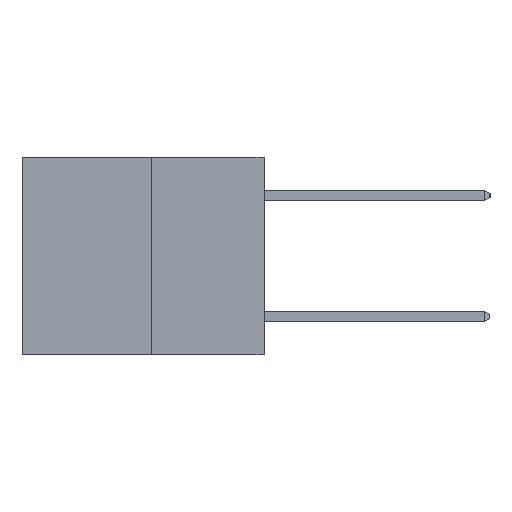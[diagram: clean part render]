
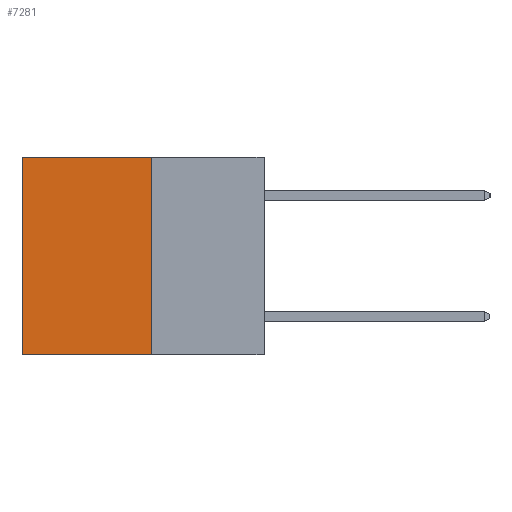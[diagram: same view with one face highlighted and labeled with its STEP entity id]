
A CAD part, left-side view. The second image highlights one B-rep face of the part: STEP entity #7281.
In plain terms, the highlighted planar face has unit normal (-1, 0, 0).
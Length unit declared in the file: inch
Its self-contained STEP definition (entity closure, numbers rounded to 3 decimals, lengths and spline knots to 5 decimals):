
#185 = CARTESIAN_POINT ( 'NONE',  ( 0.3165, 0.28, 0. ) ) ;
#335 = CARTESIAN_POINT ( 'NONE',  ( 0.3165, 0.28, -0.49 ) ) ;
#372 = DIRECTION ( 'NONE',  ( 0., 0., -1. ) ) ;
#524 = VERTEX_POINT ( 'NONE', #10380 ) ;
#536 = VECTOR ( 'NONE', #8766, 39.37008 ) ;
#1068 = DIRECTION ( 'NONE',  ( 0., 1., 0. ) ) ;
#1119 = DIRECTION ( 'NONE',  ( 1., 0., 0. ) ) ;
#1246 = ORIENTED_EDGE ( 'NONE', *, *, #8139, .T. ) ;
#1457 = VECTOR ( 'NONE', #8949, 39.37008 ) ;
#1483 = DIRECTION ( 'NONE',  ( 0., 0., -1. ) ) ;
#1568 = ORIENTED_EDGE ( 'NONE', *, *, #2744, .F. ) ;
#1746 = CARTESIAN_POINT ( 'NONE',  ( 0.3165, 0.6, -0.49 ) ) ;
#1891 = EDGE_CURVE ( 'NONE', #9267, #3325, #2910, .T. ) ;
#2524 = ORIENTED_EDGE ( 'NONE', *, *, #7141, .F. ) ;
#2616 = VECTOR ( 'NONE', #1483, 39.37008 ) ;
#2744 = EDGE_CURVE ( 'NONE', #5477, #524, #4970, .T. ) ;
#2910 = LINE ( 'NONE', #1746, #536 ) ;
#2983 = LINE ( 'NONE', #10729, #1457 ) ;
#3176 = ORIENTED_EDGE ( 'NONE', *, *, #1891, .T. ) ;
#3325 = VERTEX_POINT ( 'NONE', #9160 ) ;
#4173 = CARTESIAN_POINT ( 'NONE',  ( 0.3165, 0.28, -0.49 ) ) ;
#4711 = AXIS2_PLACEMENT_3D ( 'NONE', #335, #1119, #372 ) ;
#4819 = LINE ( 'NONE', #8121, #9346 ) ;
#4970 = LINE ( 'NONE', #4173, #2616 ) ;
#5477 = VERTEX_POINT ( 'NONE', #185 ) ;
#5588 = PLANE ( 'NONE',  #4711 ) ;
#7141 = EDGE_CURVE ( 'NONE', #524, #3325, #4819, .T. ) ;
#7281 = ADVANCED_FACE ( 'NONE', ( #8925 ), #5588, .F. ) ;
#7659 = CARTESIAN_POINT ( 'NONE',  ( 0.3165, 0.6, 0. ) ) ;
#8121 = CARTESIAN_POINT ( 'NONE',  ( 0.3165, 0.28, -0.49 ) ) ;
#8139 = EDGE_CURVE ( 'NONE', #5477, #9267, #2983, .T. ) ;
#8766 = DIRECTION ( 'NONE',  ( 0., 0., -1. ) ) ;
#8925 = FACE_OUTER_BOUND ( 'NONE', #9103, .T. ) ;
#8949 = DIRECTION ( 'NONE',  ( 0., 1., 0. ) ) ;
#9103 = EDGE_LOOP ( 'NONE', ( #3176, #2524, #1568, #1246 ) ) ;
#9160 = CARTESIAN_POINT ( 'NONE',  ( 0.3165, 0.6, -0.49 ) ) ;
#9267 = VERTEX_POINT ( 'NONE', #7659 ) ;
#9346 = VECTOR ( 'NONE', #1068, 39.37008 ) ;
#10380 = CARTESIAN_POINT ( 'NONE',  ( 0.3165, 0.28, -0.49 ) ) ;
#10729 = CARTESIAN_POINT ( 'NONE',  ( 0.3165, 0.28, 0. ) ) ;
